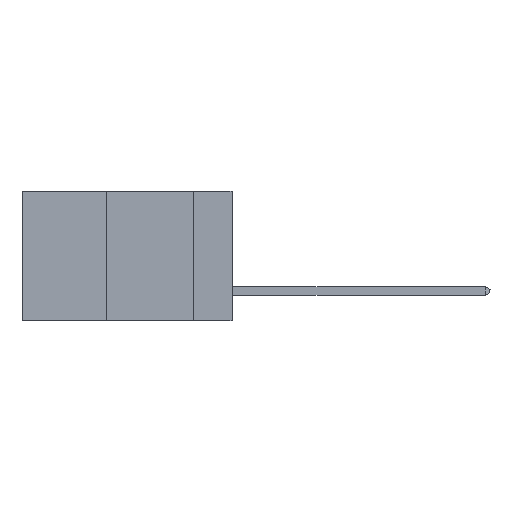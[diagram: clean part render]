
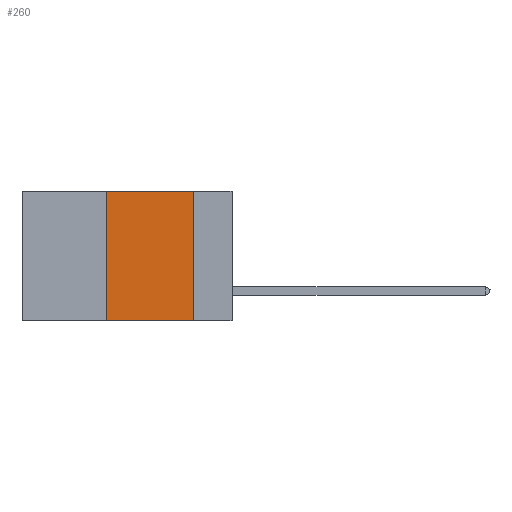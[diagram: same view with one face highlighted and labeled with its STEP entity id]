
A CAD part, left-side view. The second image highlights one B-rep face of the part: STEP entity #260.
In plain terms, the highlighted planar face has unit normal (-1, 0, 0).
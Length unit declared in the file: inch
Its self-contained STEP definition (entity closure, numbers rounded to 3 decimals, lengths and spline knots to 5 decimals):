
#260 = ADVANCED_FACE ( 'NONE', ( #8461 ), #4052, .F. ) ;
#423 = VECTOR ( 'NONE', #17801, 39.37008 ) ;
#629 = EDGE_CURVE ( 'NONE', #6174, #11948, #8962, .T. ) ;
#1017 = DIRECTION ( 'NONE',  ( 1., 0., 0. ) ) ;
#1150 = ORIENTED_EDGE ( 'NONE', *, *, #629, .T. ) ;
#1217 = VECTOR ( 'NONE', #16972, 39.37008 ) ;
#1283 = EDGE_LOOP ( 'NONE', ( #15671, #6767, #12439, #1150 ) ) ;
#1466 = VERTEX_POINT ( 'NONE', #5795 ) ;
#2597 = VERTEX_POINT ( 'NONE', #12470 ) ;
#2715 = LINE ( 'NONE', #10398, #423 ) ;
#2807 = EDGE_CURVE ( 'NONE', #6174, #1466, #2715, .T. ) ;
#4052 = PLANE ( 'NONE',  #6465 ) ;
#5795 = CARTESIAN_POINT ( 'NONE',  ( 0., 0.36, 0. ) ) ;
#6174 = VERTEX_POINT ( 'NONE', #15321 ) ;
#6465 = AXIS2_PLACEMENT_3D ( 'NONE', #8385, #1017, #18378 ) ;
#6767 = ORIENTED_EDGE ( 'NONE', *, *, #18372, .F. ) ;
#8219 = DIRECTION ( 'NONE',  ( 0., 0., -1. ) ) ;
#8385 = CARTESIAN_POINT ( 'NONE',  ( 0., 0.6, 0. ) ) ;
#8461 = FACE_OUTER_BOUND ( 'NONE', #1283, .T. ) ;
#8962 = LINE ( 'NONE', #14127, #1217 ) ;
#9997 = VECTOR ( 'NONE', #15422, 39.37008 ) ;
#10398 = CARTESIAN_POINT ( 'NONE',  ( 0., 0.36, 0. ) ) ;
#10703 = EDGE_CURVE ( 'NONE', #2597, #11948, #12305, .T. ) ;
#10913 = LINE ( 'NONE', #11122, #9997 ) ;
#11122 = CARTESIAN_POINT ( 'NONE',  ( 0., 0.6, 0. ) ) ;
#11948 = VERTEX_POINT ( 'NONE', #14190 ) ;
#12305 = LINE ( 'NONE', #15432, #13643 ) ;
#12439 = ORIENTED_EDGE ( 'NONE', *, *, #2807, .F. ) ;
#12470 = CARTESIAN_POINT ( 'NONE',  ( 0., 0.11, 0. ) ) ;
#13643 = VECTOR ( 'NONE', #8219, 39.37008 ) ;
#14127 = CARTESIAN_POINT ( 'NONE',  ( 0., 0.6, -0.37 ) ) ;
#14190 = CARTESIAN_POINT ( 'NONE',  ( 0., 0.11, -0.37 ) ) ;
#15321 = CARTESIAN_POINT ( 'NONE',  ( 0., 0.36, -0.37 ) ) ;
#15422 = DIRECTION ( 'NONE',  ( 0., -1., 0. ) ) ;
#15432 = CARTESIAN_POINT ( 'NONE',  ( 0., 0.11, 0. ) ) ;
#15671 = ORIENTED_EDGE ( 'NONE', *, *, #10703, .F. ) ;
#16972 = DIRECTION ( 'NONE',  ( 0., -1., 0. ) ) ;
#17801 = DIRECTION ( 'NONE',  ( 0., 0., 1. ) ) ;
#18372 = EDGE_CURVE ( 'NONE', #1466, #2597, #10913, .T. ) ;
#18378 = DIRECTION ( 'NONE',  ( 0., 0., -1. ) ) ;
